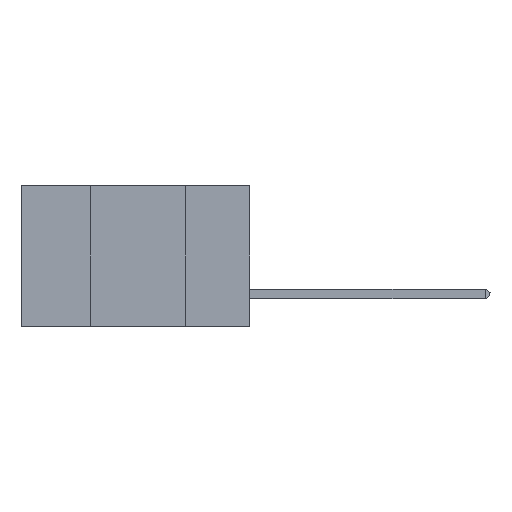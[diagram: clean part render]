
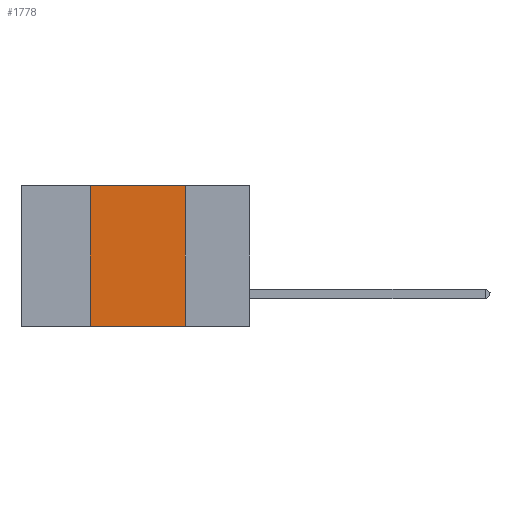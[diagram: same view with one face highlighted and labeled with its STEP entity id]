
A CAD part, left-side view. The second image highlights one B-rep face of the part: STEP entity #1778.
In plain terms, the highlighted planar face has unit normal (-1, 0, 0).
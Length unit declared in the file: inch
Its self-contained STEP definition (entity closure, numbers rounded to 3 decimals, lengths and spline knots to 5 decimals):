
#62 = VECTOR ( 'NONE', #8825, 39.37008 ) ;
#591 = EDGE_LOOP ( 'NONE', ( #12372, #11773, #8063, #7246 ) ) ;
#1180 = VERTEX_POINT ( 'NONE', #1712 ) ;
#1544 = VERTEX_POINT ( 'NONE', #9295 ) ;
#1712 = CARTESIAN_POINT ( 'NONE',  ( 0., 0.17, -0.37 ) ) ;
#1778 = ADVANCED_FACE ( 'NONE', ( #3023 ), #8437, .F. ) ;
#2062 = AXIS2_PLACEMENT_3D ( 'NONE', #4231, #8610, #10079 ) ;
#2384 = VECTOR ( 'NONE', #16568, 39.37008 ) ;
#2487 = EDGE_CURVE ( 'NONE', #14112, #14838, #3645, .T. ) ;
#3023 = FACE_OUTER_BOUND ( 'NONE', #591, .T. ) ;
#3645 = LINE ( 'NONE', #16820, #8872 ) ;
#4136 = VECTOR ( 'NONE', #11329, 39.37008 ) ;
#4231 = CARTESIAN_POINT ( 'NONE',  ( 0., 0.6, 0. ) ) ;
#5547 = LINE ( 'NONE', #16002, #62 ) ;
#7002 = CARTESIAN_POINT ( 'NONE',  ( 0., 0.17, 0. ) ) ;
#7246 = ORIENTED_EDGE ( 'NONE', *, *, #14310, .T. ) ;
#8009 = CARTESIAN_POINT ( 'NONE',  ( 0., 0.42, 0. ) ) ;
#8063 = ORIENTED_EDGE ( 'NONE', *, *, #12132, .F. ) ;
#8437 = PLANE ( 'NONE',  #2062 ) ;
#8513 = DIRECTION ( 'NONE',  ( 0., -1., 0. ) ) ;
#8610 = DIRECTION ( 'NONE',  ( 1., 0., 0. ) ) ;
#8825 = DIRECTION ( 'NONE',  ( 0., -1., 0. ) ) ;
#8872 = VECTOR ( 'NONE', #8513, 39.37008 ) ;
#9295 = CARTESIAN_POINT ( 'NONE',  ( 0., 0.42, -0.37 ) ) ;
#10079 = DIRECTION ( 'NONE',  ( 0., 0., -1. ) ) ;
#11329 = DIRECTION ( 'NONE',  ( 0., 0., -1. ) ) ;
#11480 = EDGE_CURVE ( 'NONE', #14838, #1180, #12057, .T. ) ;
#11773 = ORIENTED_EDGE ( 'NONE', *, *, #2487, .F. ) ;
#12057 = LINE ( 'NONE', #7002, #4136 ) ;
#12132 = EDGE_CURVE ( 'NONE', #1544, #14112, #15999, .T. ) ;
#12292 = CARTESIAN_POINT ( 'NONE',  ( 0., 0.42, 0. ) ) ;
#12372 = ORIENTED_EDGE ( 'NONE', *, *, #11480, .F. ) ;
#13884 = CARTESIAN_POINT ( 'NONE',  ( 0., 0.17, 0. ) ) ;
#14112 = VERTEX_POINT ( 'NONE', #12292 ) ;
#14310 = EDGE_CURVE ( 'NONE', #1544, #1180, #5547, .T. ) ;
#14838 = VERTEX_POINT ( 'NONE', #13884 ) ;
#15999 = LINE ( 'NONE', #8009, #2384 ) ;
#16002 = CARTESIAN_POINT ( 'NONE',  ( 0., 0.6, -0.37 ) ) ;
#16568 = DIRECTION ( 'NONE',  ( 0., 0., 1. ) ) ;
#16820 = CARTESIAN_POINT ( 'NONE',  ( 0., 0.6, 0. ) ) ;
